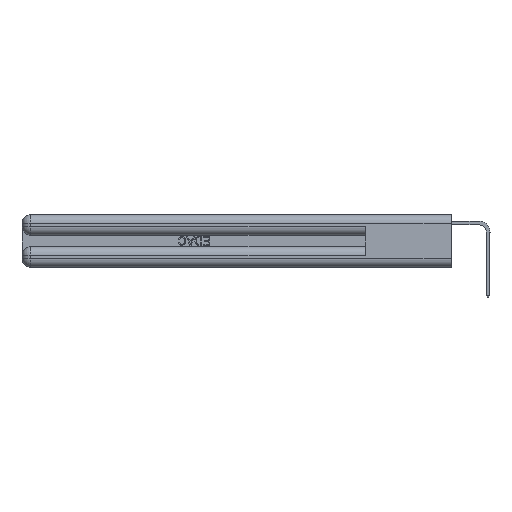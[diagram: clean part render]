
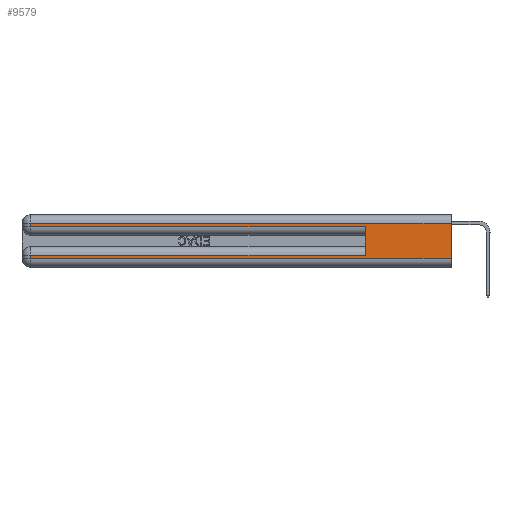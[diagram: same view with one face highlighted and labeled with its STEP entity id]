
A CAD part, left-side view. The second image highlights one B-rep face of the part: STEP entity #9579.
In plain terms, the highlighted planar face has unit normal (-1, 0, 0).
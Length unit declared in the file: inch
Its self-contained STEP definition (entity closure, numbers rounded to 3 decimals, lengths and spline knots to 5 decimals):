
#110 = VERTEX_POINT ( 'NONE', #19507 ) ;
#2158 = CARTESIAN_POINT ( 'NONE',  ( 0., 0., 0.06 ) ) ;
#2255 = CARTESIAN_POINT ( 'NONE',  ( 0., 2.94, 0.37 ) ) ;
#2703 = DIRECTION ( 'NONE',  ( 0., 0., -1. ) ) ;
#3262 = DIRECTION ( 'NONE',  ( 0., 0., 1. ) ) ;
#3881 = FACE_OUTER_BOUND ( 'NONE', #17568, .T. ) ;
#3917 = VECTOR ( 'NONE', #26408, 39.37008 ) ;
#4041 = LINE ( 'NONE', #2158, #16864 ) ;
#4765 = DIRECTION ( 'NONE',  ( 0., -1., 0. ) ) ;
#4831 = ORIENTED_EDGE ( 'NONE', *, *, #22042, .T. ) ;
#5163 = LINE ( 'NONE', #25682, #19542 ) ;
#5383 = EDGE_CURVE ( 'NONE', #110, #16302, #22392, .T. ) ;
#5384 = VERTEX_POINT ( 'NONE', #30447 ) ;
#5434 = VERTEX_POINT ( 'NONE', #8047 ) ;
#6196 = LINE ( 'NONE', #23645, #18946 ) ;
#7294 = ORIENTED_EDGE ( 'NONE', *, *, #16299, .T. ) ;
#7320 = DIRECTION ( 'NONE',  ( 0., 1., 0. ) ) ;
#7624 = CARTESIAN_POINT ( 'NONE',  ( 0., 0.6, 0.085 ) ) ;
#8047 = CARTESIAN_POINT ( 'NONE',  ( 0., 0.6, 0.285 ) ) ;
#8696 = CARTESIAN_POINT ( 'NONE',  ( 0., 0., 0.37 ) ) ;
#8751 = CARTESIAN_POINT ( 'NONE',  ( 0., 0., 0.06 ) ) ;
#8923 = VERTEX_POINT ( 'NONE', #20808 ) ;
#9313 = LINE ( 'NONE', #17655, #28592 ) ;
#9579 = ADVANCED_FACE ( 'NONE', ( #3881 ), #26359, .F. ) ;
#9667 = CARTESIAN_POINT ( 'NONE',  ( 0., 0., 0.285 ) ) ;
#9944 = AXIS2_PLACEMENT_3D ( 'NONE', #8696, #11263, #28840 ) ;
#10566 = DIRECTION ( 'NONE',  ( 0., 1., 0. ) ) ;
#11263 = DIRECTION ( 'NONE',  ( 1., 0., 0. ) ) ;
#11285 = EDGE_CURVE ( 'NONE', #21243, #5434, #6196, .T. ) ;
#12458 = ORIENTED_EDGE ( 'NONE', *, *, #15851, .T. ) ;
#13287 = ORIENTED_EDGE ( 'NONE', *, *, #20553, .T. ) ;
#13921 = VERTEX_POINT ( 'NONE', #19960 ) ;
#14878 = ORIENTED_EDGE ( 'NONE', *, *, #27275, .T. ) ;
#15851 = EDGE_CURVE ( 'NONE', #5384, #5434, #24241, .T. ) ;
#16299 = EDGE_CURVE ( 'NONE', #8923, #13921, #29999, .T. ) ;
#16302 = VERTEX_POINT ( 'NONE', #8751 ) ;
#16864 = VECTOR ( 'NONE', #4765, 39.37008 ) ;
#17568 = EDGE_LOOP ( 'NONE', ( #24310, #4831, #31651, #12458, #19217, #13287, #7294, #14878 ) ) ;
#17655 = CARTESIAN_POINT ( 'NONE',  ( 0., 0., 0.085 ) ) ;
#18040 = CARTESIAN_POINT ( 'NONE',  ( 0., 0., 0.37 ) ) ;
#18856 = CARTESIAN_POINT ( 'NONE',  ( 0., 2.94, 0.37 ) ) ;
#18870 = VERTEX_POINT ( 'NONE', #31574 ) ;
#18946 = VECTOR ( 'NONE', #3262, 39.37008 ) ;
#19217 = ORIENTED_EDGE ( 'NONE', *, *, #11285, .F. ) ;
#19507 = CARTESIAN_POINT ( 'NONE',  ( 0., 0., 0.31 ) ) ;
#19542 = VECTOR ( 'NONE', #10566, 39.37008 ) ;
#19714 = EDGE_CURVE ( 'NONE', #18870, #5384, #27094, .T. ) ;
#19960 = CARTESIAN_POINT ( 'NONE',  ( 0., 2.94, 0.06 ) ) ;
#20476 = VECTOR ( 'NONE', #30124, 39.37008 ) ;
#20553 = EDGE_CURVE ( 'NONE', #21243, #8923, #9313, .T. ) ;
#20808 = CARTESIAN_POINT ( 'NONE',  ( 0., 2.94, 0.085 ) ) ;
#21243 = VERTEX_POINT ( 'NONE', #7624 ) ;
#21603 = VECTOR ( 'NONE', #2703, 39.37008 ) ;
#22042 = EDGE_CURVE ( 'NONE', #110, #18870, #5163, .T. ) ;
#22392 = LINE ( 'NONE', #18040, #21603 ) ;
#23645 = CARTESIAN_POINT ( 'NONE',  ( 0., 0.6, 0.145 ) ) ;
#24241 = LINE ( 'NONE', #9667, #30030 ) ;
#24310 = ORIENTED_EDGE ( 'NONE', *, *, #5383, .F. ) ;
#24797 = DIRECTION ( 'NONE',  ( 0., -1., 0. ) ) ;
#25682 = CARTESIAN_POINT ( 'NONE',  ( 0., 0., 0.31 ) ) ;
#26359 = PLANE ( 'NONE',  #9944 ) ;
#26408 = DIRECTION ( 'NONE',  ( 0., 0., -1. ) ) ;
#27094 = LINE ( 'NONE', #2255, #20476 ) ;
#27275 = EDGE_CURVE ( 'NONE', #13921, #16302, #4041, .T. ) ;
#28592 = VECTOR ( 'NONE', #7320, 39.37008 ) ;
#28840 = DIRECTION ( 'NONE',  ( 0., 0., -1. ) ) ;
#29999 = LINE ( 'NONE', #18856, #3917 ) ;
#30030 = VECTOR ( 'NONE', #24797, 39.37008 ) ;
#30124 = DIRECTION ( 'NONE',  ( 0., 0., -1. ) ) ;
#30447 = CARTESIAN_POINT ( 'NONE',  ( 0., 2.94, 0.285 ) ) ;
#31574 = CARTESIAN_POINT ( 'NONE',  ( 0., 2.94, 0.31 ) ) ;
#31651 = ORIENTED_EDGE ( 'NONE', *, *, #19714, .T. ) ;
